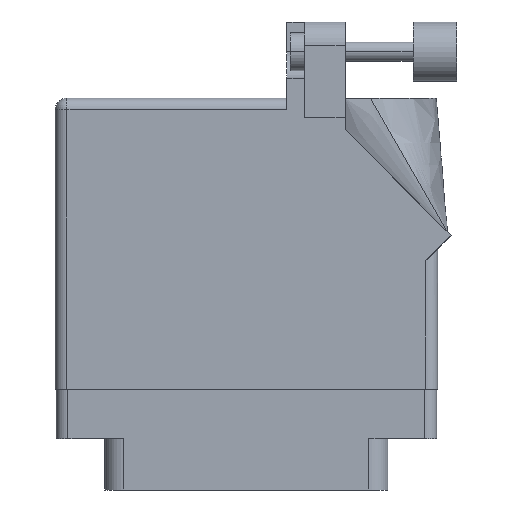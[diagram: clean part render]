
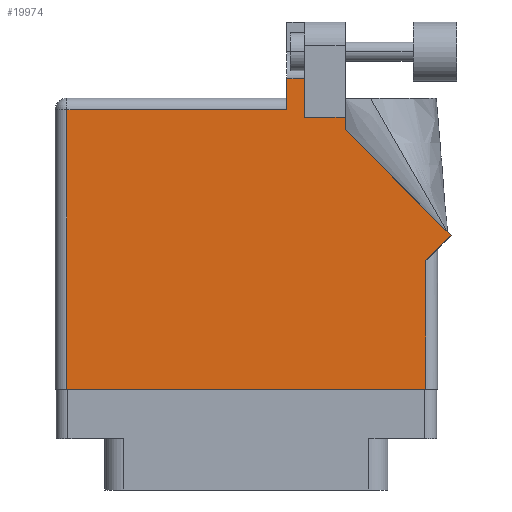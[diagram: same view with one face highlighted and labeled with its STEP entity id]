
A CAD part, front view. The second image highlights one B-rep face of the part: STEP entity #19974.
In plain terms, the highlighted face is planar.
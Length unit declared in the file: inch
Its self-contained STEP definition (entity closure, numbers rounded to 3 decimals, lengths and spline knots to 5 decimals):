
#89 = VERTEX_POINT ( 'NONE', #11617 ) ;
#575 = CARTESIAN_POINT ( 'NONE',  ( 1.311, 1.6315, 0. ) ) ;
#640 = CARTESIAN_POINT ( 'NONE',  ( 2.08071, 0.80771, 0. ) ) ;
#676 = DIRECTION ( 'NONE',  ( -1., 0., 0. ) ) ;
#839 = LINE ( 'NONE', #10711, #6899 ) ;
#1071 = VERTEX_POINT ( 'NONE', #1373 ) ;
#1206 = EDGE_CURVE ( 'NONE', #7749, #89, #16464, .T. ) ;
#1373 = CARTESIAN_POINT ( 'NONE',  ( 2.08071, 0.80771, 0. ) ) ;
#1429 = EDGE_CURVE ( 'NONE', #89, #15953, #6992, .T. ) ;
#1756 = LINE ( 'NONE', #18882, #7441 ) ;
#1826 = EDGE_CURVE ( 'NONE', #11412, #14024, #7713, .T. ) ;
#2861 = LINE ( 'NONE', #25912, #14260 ) ;
#3076 = ORIENTED_EDGE ( 'NONE', *, *, #19024, .T. ) ;
#3252 = CARTESIAN_POINT ( 'NONE',  ( 0., 0., 0. ) ) ;
#3457 = CARTESIAN_POINT ( 'NONE',  ( 0., 1.468, 0. ) ) ;
#4017 = AXIS2_PLACEMENT_3D ( 'NONE', #26584, #24159, #21600 ) ;
#4282 = ORIENTED_EDGE ( 'NONE', *, *, #29602, .T. ) ;
#4601 = PLANE ( 'NONE',  #4017 ) ;
#5024 = CARTESIAN_POINT ( 'NONE',  ( 1.524, 1.36442, 0. ) ) ;
#5720 = CARTESIAN_POINT ( 'NONE',  ( 1.311, 1.43, 0. ) ) ;
#6263 = LINE ( 'NONE', #9811, #24503 ) ;
#6571 = CARTESIAN_POINT ( 'NONE',  ( 1.948, 0., 0. ) ) ;
#6878 = EDGE_CURVE ( 'NONE', #28287, #11412, #23464, .T. ) ;
#6899 = VECTOR ( 'NONE', #10918, 39.37008 ) ;
#6992 = LINE ( 'NONE', #3457, #21423 ) ;
#7003 = LINE ( 'NONE', #640, #30908 ) ;
#7441 = VECTOR ( 'NONE', #23655, 39.37008 ) ;
#7509 = LINE ( 'NONE', #12231, #31435 ) ;
#7713 = LINE ( 'NONE', #19360, #21764 ) ;
#7749 = VERTEX_POINT ( 'NONE', #24316 ) ;
#8048 = DIRECTION ( 'NONE',  ( 1., 0., 0. ) ) ;
#8090 = VERTEX_POINT ( 'NONE', #5720 ) ;
#8127 = CARTESIAN_POINT ( 'NONE',  ( 0.062, 0., 0. ) ) ;
#9588 = ORIENTED_EDGE ( 'NONE', *, *, #6878, .T. ) ;
#9811 = CARTESIAN_POINT ( 'NONE',  ( 1.311, 1.43, 0. ) ) ;
#10574 = ORIENTED_EDGE ( 'NONE', *, *, #12844, .T. ) ;
#10711 = CARTESIAN_POINT ( 'NONE',  ( 1.524, 1.36442, 0. ) ) ;
#10918 = DIRECTION ( 'NONE',  ( 0., 1., 0. ) ) ;
#11073 = EDGE_CURVE ( 'NONE', #15953, #28287, #7509, .T. ) ;
#11412 = VERTEX_POINT ( 'NONE', #6571 ) ;
#11575 = VERTEX_POINT ( 'NONE', #29231 ) ;
#11617 = CARTESIAN_POINT ( 'NONE',  ( 1.217, 1.468, 0. ) ) ;
#12184 = CARTESIAN_POINT ( 'NONE',  ( 1.217, 1.53, 0. ) ) ;
#12231 = CARTESIAN_POINT ( 'NONE',  ( 0.062, 0., 0. ) ) ;
#12844 = EDGE_CURVE ( 'NONE', #8090, #13838, #6263, .T. ) ;
#12937 = ORIENTED_EDGE ( 'NONE', *, *, #1826, .T. ) ;
#13015 = CARTESIAN_POINT ( 'NONE',  ( 1.524, 1.43, 0. ) ) ;
#13838 = VERTEX_POINT ( 'NONE', #575 ) ;
#13962 = ORIENTED_EDGE ( 'NONE', *, *, #1429, .T. ) ;
#14024 = VERTEX_POINT ( 'NONE', #17004 ) ;
#14260 = VECTOR ( 'NONE', #20796, 39.37008 ) ;
#14593 = ORIENTED_EDGE ( 'NONE', *, *, #17414, .T. ) ;
#15953 = VERTEX_POINT ( 'NONE', #27329 ) ;
#16464 = LINE ( 'NONE', #12184, #24838 ) ;
#17004 = CARTESIAN_POINT ( 'NONE',  ( 1.948, 0.675, 0. ) ) ;
#17414 = EDGE_CURVE ( 'NONE', #11575, #8090, #20399, .T. ) ;
#17439 = DIRECTION ( 'NONE',  ( -0.707, 0.707, 0. ) ) ;
#18882 = CARTESIAN_POINT ( 'NONE',  ( 1.64177, 1.6315, 0. ) ) ;
#19024 = EDGE_CURVE ( 'NONE', #1071, #30507, #7003, .T. ) ;
#19273 = VECTOR ( 'NONE', #8048, 39.37008 ) ;
#19360 = CARTESIAN_POINT ( 'NONE',  ( 1.948, 0.737, 0. ) ) ;
#19974 = ADVANCED_FACE ( 'NONE', ( #25174 ), #4601, .F. ) ;
#20048 = ORIENTED_EDGE ( 'NONE', *, *, #26293, .T. ) ;
#20174 = ORIENTED_EDGE ( 'NONE', *, *, #1206, .T. ) ;
#20399 = LINE ( 'NONE', #13015, #27257 ) ;
#20796 = DIRECTION ( 'NONE',  ( 0.707, 0.707, 0. ) ) ;
#21423 = VECTOR ( 'NONE', #23108, 39.37008 ) ;
#21600 = DIRECTION ( 'NONE',  ( -1., 0., 0. ) ) ;
#21764 = VECTOR ( 'NONE', #26785, 39.37008 ) ;
#22251 = EDGE_CURVE ( 'NONE', #30507, #11575, #839, .T. ) ;
#23108 = DIRECTION ( 'NONE',  ( -1., 0., 0. ) ) ;
#23183 = ORIENTED_EDGE ( 'NONE', *, *, #11073, .T. ) ;
#23464 = LINE ( 'NONE', #3252, #19273 ) ;
#23655 = DIRECTION ( 'NONE',  ( -1., 0., 0. ) ) ;
#24159 = DIRECTION ( 'NONE',  ( 0., 0., -1. ) ) ;
#24192 = DIRECTION ( 'NONE',  ( 0., -1., 0. ) ) ;
#24316 = CARTESIAN_POINT ( 'NONE',  ( 1.217, 1.6315, 0. ) ) ;
#24503 = VECTOR ( 'NONE', #26786, 39.37008 ) ;
#24727 = ORIENTED_EDGE ( 'NONE', *, *, #22251, .T. ) ;
#24838 = VECTOR ( 'NONE', #24192, 39.37008 ) ;
#25174 = FACE_OUTER_BOUND ( 'NONE', #27728, .T. ) ;
#25912 = CARTESIAN_POINT ( 'NONE',  ( 2.01, 0.737, 0. ) ) ;
#26293 = EDGE_CURVE ( 'NONE', #14024, #1071, #2861, .T. ) ;
#26584 = CARTESIAN_POINT ( 'NONE',  ( 0., 1.53, 0. ) ) ;
#26785 = DIRECTION ( 'NONE',  ( 0., 1., 0. ) ) ;
#26786 = DIRECTION ( 'NONE',  ( 0., 1., 0. ) ) ;
#27081 = DIRECTION ( 'NONE',  ( 0., -1., 0. ) ) ;
#27257 = VECTOR ( 'NONE', #676, 39.37008 ) ;
#27329 = CARTESIAN_POINT ( 'NONE',  ( 0.062, 1.468, 0. ) ) ;
#27728 = EDGE_LOOP ( 'NONE', ( #10574, #4282, #20174, #13962, #23183, #9588, #12937, #20048, #3076, #24727, #14593 ) ) ;
#28287 = VERTEX_POINT ( 'NONE', #8127 ) ;
#29231 = CARTESIAN_POINT ( 'NONE',  ( 1.524, 1.43, 0. ) ) ;
#29602 = EDGE_CURVE ( 'NONE', #13838, #7749, #1756, .T. ) ;
#30507 = VERTEX_POINT ( 'NONE', #5024 ) ;
#30908 = VECTOR ( 'NONE', #17439, 39.37008 ) ;
#31435 = VECTOR ( 'NONE', #27081, 39.37008 ) ;
